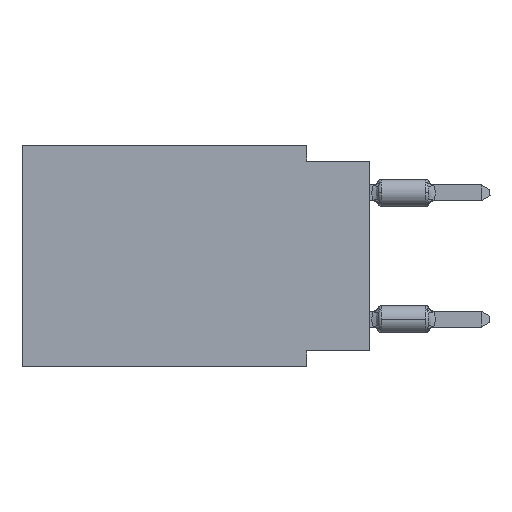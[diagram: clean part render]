
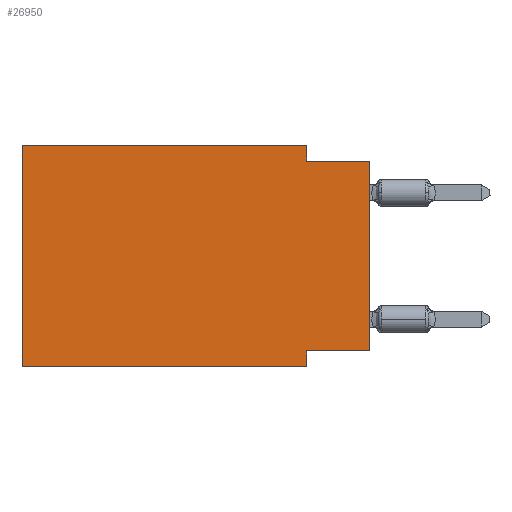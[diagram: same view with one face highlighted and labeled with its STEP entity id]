
A CAD part, left-side view. The second image highlights one B-rep face of the part: STEP entity #26950.
In plain terms, the highlighted planar face has unit normal (-1, 0, 0).
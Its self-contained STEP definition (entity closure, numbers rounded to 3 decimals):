
#352 = CARTESIAN_POINT ( 'NONE',  ( 0., 2.54, 0. ) ) ;
#535 = VERTEX_POINT ( 'NONE', #352 ) ;
#1642 = VECTOR ( 'NONE', #15667, 1000. ) ;
#1725 = ORIENTED_EDGE ( 'NONE', *, *, #26318, .F. ) ;
#2035 = EDGE_CURVE ( 'NONE', #17695, #3275, #43075, .T. ) ;
#2560 = CARTESIAN_POINT ( 'NONE',  ( 0., 2.54, 0. ) ) ;
#2964 = VERTEX_POINT ( 'NONE', #22414 ) ;
#3172 = ORIENTED_EDGE ( 'NONE', *, *, #2035, .F. ) ;
#3275 = VERTEX_POINT ( 'NONE', #20640 ) ;
#3709 = ORIENTED_EDGE ( 'NONE', *, *, #20641, .F. ) ;
#3754 = DIRECTION ( 'NONE',  ( 0., -1., 0. ) ) ;
#4505 = DIRECTION ( 'NONE',  ( 0., 0., -1. ) ) ;
#7525 = EDGE_LOOP ( 'NONE', ( #17339, #36163, #35070, #3709, #3172, #36033, #37833, #1725 ) ) ;
#7720 = EDGE_CURVE ( 'NONE', #17695, #2964, #14710, .T. ) ;
#7764 = VERTEX_POINT ( 'NONE', #33394 ) ;
#7964 = CARTESIAN_POINT ( 'NONE',  ( 0., 0., -0.635 ) ) ;
#8260 = CARTESIAN_POINT ( 'NONE',  ( 0., 2.54, -8.89 ) ) ;
#12491 = LINE ( 'NONE', #8260, #30431 ) ;
#12534 = DIRECTION ( 'NONE',  ( 0., 0., -1. ) ) ;
#12884 = CARTESIAN_POINT ( 'NONE',  ( 0., 2.54, -8.255 ) ) ;
#14710 = LINE ( 'NONE', #30657, #47219 ) ;
#15350 = CARTESIAN_POINT ( 'NONE',  ( 0., 13.97, 0. ) ) ;
#15667 = DIRECTION ( 'NONE',  ( 0., -1., 0. ) ) ;
#16925 = LINE ( 'NONE', #21186, #43407 ) ;
#17135 = CARTESIAN_POINT ( 'NONE',  ( 0., 2.54, -0.635 ) ) ;
#17339 = ORIENTED_EDGE ( 'NONE', *, *, #30193, .T. ) ;
#17695 = VERTEX_POINT ( 'NONE', #38416 ) ;
#17802 = DIRECTION ( 'NONE',  ( 0., 0., -1. ) ) ;
#18301 = VECTOR ( 'NONE', #3754, 1000. ) ;
#18697 = DIRECTION ( 'NONE',  ( 0., -1., 0. ) ) ;
#18912 = LINE ( 'NONE', #46091, #29053 ) ;
#18981 = CARTESIAN_POINT ( 'NONE',  ( 0., 13.97, 0. ) ) ;
#19092 = DIRECTION ( 'NONE',  ( 1., 0., 0. ) ) ;
#20640 = CARTESIAN_POINT ( 'NONE',  ( 0., 13.97, 0. ) ) ;
#20641 = EDGE_CURVE ( 'NONE', #3275, #535, #30698, .T. ) ;
#21186 = CARTESIAN_POINT ( 'NONE',  ( 0., 0., -8.255 ) ) ;
#22264 = EDGE_CURVE ( 'NONE', #30482, #36310, #25191, .T. ) ;
#22414 = CARTESIAN_POINT ( 'NONE',  ( 0., 2.54, -8.89 ) ) ;
#23049 = VECTOR ( 'NONE', #43809, 1000. ) ;
#25061 = LINE ( 'NONE', #2560, #46666 ) ;
#25191 = LINE ( 'NONE', #46100, #1642 ) ;
#26318 = EDGE_CURVE ( 'NONE', #7764, #39353, #16925, .T. ) ;
#26950 = ADVANCED_FACE ( 'NONE', ( #46958 ), #34042, .F. ) ;
#29053 = VECTOR ( 'NONE', #34101, 1000. ) ;
#29089 = AXIS2_PLACEMENT_3D ( 'NONE', #15350, #19092, #12534 ) ;
#30193 = EDGE_CURVE ( 'NONE', #7764, #36310, #18912, .T. ) ;
#30431 = VECTOR ( 'NONE', #4505, 1000. ) ;
#30482 = VERTEX_POINT ( 'NONE', #17135 ) ;
#30657 = CARTESIAN_POINT ( 'NONE',  ( 0., 13.97, -8.89 ) ) ;
#30698 = LINE ( 'NONE', #18981, #18301 ) ;
#33276 = EDGE_CURVE ( 'NONE', #39353, #2964, #12491, .T. ) ;
#33394 = CARTESIAN_POINT ( 'NONE',  ( 0., 0., -8.255 ) ) ;
#34042 = PLANE ( 'NONE',  #29089 ) ;
#34101 = DIRECTION ( 'NONE',  ( 0., 0., 1. ) ) ;
#35070 = ORIENTED_EDGE ( 'NONE', *, *, #46188, .F. ) ;
#36033 = ORIENTED_EDGE ( 'NONE', *, *, #7720, .T. ) ;
#36163 = ORIENTED_EDGE ( 'NONE', *, *, #22264, .F. ) ;
#36310 = VERTEX_POINT ( 'NONE', #7964 ) ;
#37833 = ORIENTED_EDGE ( 'NONE', *, *, #33276, .F. ) ;
#38416 = CARTESIAN_POINT ( 'NONE',  ( 0., 13.97, -8.89 ) ) ;
#39353 = VERTEX_POINT ( 'NONE', #12884 ) ;
#43075 = LINE ( 'NONE', #46834, #23049 ) ;
#43407 = VECTOR ( 'NONE', #46891, 1000. ) ;
#43809 = DIRECTION ( 'NONE',  ( 0., 0., 1. ) ) ;
#46091 = CARTESIAN_POINT ( 'NONE',  ( 0., 0., 0. ) ) ;
#46100 = CARTESIAN_POINT ( 'NONE',  ( 0., 0., -0.635 ) ) ;
#46188 = EDGE_CURVE ( 'NONE', #535, #30482, #25061, .T. ) ;
#46666 = VECTOR ( 'NONE', #17802, 1000. ) ;
#46834 = CARTESIAN_POINT ( 'NONE',  ( 0., 13.97, 0. ) ) ;
#46891 = DIRECTION ( 'NONE',  ( 0., 1., 0. ) ) ;
#46958 = FACE_OUTER_BOUND ( 'NONE', #7525, .T. ) ;
#47219 = VECTOR ( 'NONE', #18697, 1000. ) ;
